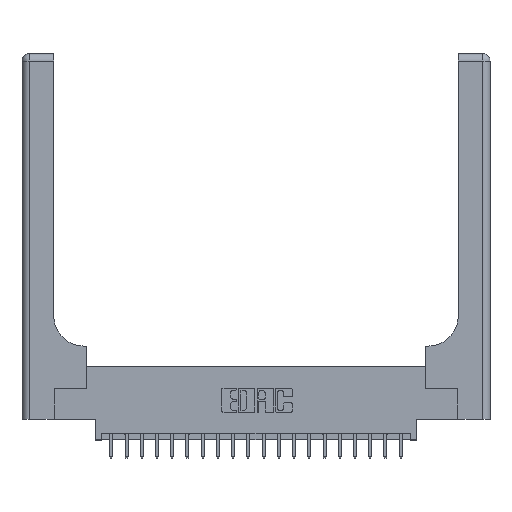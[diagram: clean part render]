
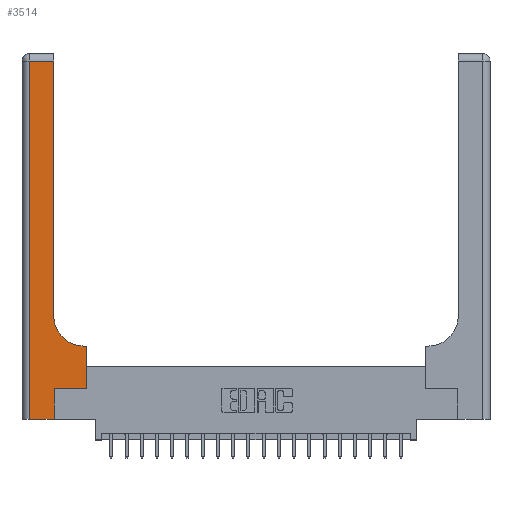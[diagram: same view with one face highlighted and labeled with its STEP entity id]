
A CAD part, top view. The second image highlights one B-rep face of the part: STEP entity #3514.
In plain terms, the highlighted planar face has unit normal (0, 0, 1).
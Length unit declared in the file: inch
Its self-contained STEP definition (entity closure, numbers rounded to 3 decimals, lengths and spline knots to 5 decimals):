
#363 = CARTESIAN_POINT ( 'NONE',  ( 0., 0., 0.37 ) ) ;
#433 = EDGE_CURVE ( 'NONE', #7438, #18347, #4337, .T. ) ;
#518 = EDGE_LOOP ( 'NONE', ( #19080, #19223, #4699, #2922, #15603, #11570, #15642, #14429, #13292 ) ) ;
#813 = EDGE_CURVE ( 'NONE', #16541, #18114, #10615, .T. ) ;
#1214 = CARTESIAN_POINT ( 'NONE',  ( 0.265, 0., 0.37 ) ) ;
#1371 = DIRECTION ( 'NONE',  ( 0., 0., -1. ) ) ;
#1857 = CARTESIAN_POINT ( 'NONE',  ( 0.528, 0.6, 0.37 ) ) ;
#1941 = EDGE_CURVE ( 'NONE', #14436, #12243, #16489, .T. ) ;
#1986 = EDGE_CURVE ( 'NONE', #7854, #16624, #10456, .T. ) ;
#1988 = AXIS2_PLACEMENT_3D ( 'NONE', #18352, #1371, #18024 ) ;
#2592 = PLANE ( 'NONE',  #16197 ) ;
#2777 = EDGE_CURVE ( 'NONE', #16624, #7438, #20082, .T. ) ;
#2892 = LINE ( 'NONE', #9523, #16131 ) ;
#2922 = ORIENTED_EDGE ( 'NONE', *, *, #813, .T. ) ;
#3074 = CARTESIAN_POINT ( 'NONE',  ( 0.26, 0.85, 0.37 ) ) ;
#3514 = ADVANCED_FACE ( 'NONE', ( #15956 ), #2592, .F. ) ;
#3978 = EDGE_CURVE ( 'NONE', #12243, #4757, #8069, .T. ) ;
#4292 = CARTESIAN_POINT ( 'NONE',  ( 0.06, 0., 0.37 ) ) ;
#4337 = LINE ( 'NONE', #7555, #20530 ) ;
#4699 = ORIENTED_EDGE ( 'NONE', *, *, #10388, .T. ) ;
#4757 = VERTEX_POINT ( 'NONE', #1857 ) ;
#5111 = LINE ( 'NONE', #18792, #20219 ) ;
#6352 = VECTOR ( 'NONE', #14799, 39.37008 ) ;
#7398 = LINE ( 'NONE', #17109, #15805 ) ;
#7438 = VERTEX_POINT ( 'NONE', #7890 ) ;
#7555 = CARTESIAN_POINT ( 'NONE',  ( 0., 2.94, 0.37 ) ) ;
#7854 = VERTEX_POINT ( 'NONE', #18119 ) ;
#7890 = CARTESIAN_POINT ( 'NONE',  ( 0.26, 2.94, 0.37 ) ) ;
#8069 = LINE ( 'NONE', #19318, #6352 ) ;
#8298 = EDGE_CURVE ( 'NONE', #18114, #14436, #7398, .T. ) ;
#8405 = VECTOR ( 'NONE', #13152, 39.37008 ) ;
#9523 = CARTESIAN_POINT ( 'NONE',  ( 0.26, 0.6, 0.37 ) ) ;
#9726 = CARTESIAN_POINT ( 'NONE',  ( 0.26, 3., 0.37 ) ) ;
#10388 = EDGE_CURVE ( 'NONE', #18347, #16541, #5111, .T. ) ;
#10391 = DIRECTION ( 'NONE',  ( 0., 1., 0. ) ) ;
#10456 = CIRCLE ( 'NONE', #1988, 0.25 ) ;
#10615 = LINE ( 'NONE', #363, #15276 ) ;
#11570 = ORIENTED_EDGE ( 'NONE', *, *, #1941, .T. ) ;
#12243 = VERTEX_POINT ( 'NONE', #19852 ) ;
#12337 = CARTESIAN_POINT ( 'NONE',  ( 0.265, 0.25, 0.37 ) ) ;
#12849 = DIRECTION ( 'NONE',  ( -1., 0., 0. ) ) ;
#13070 = DIRECTION ( 'NONE',  ( 1., 0., 0. ) ) ;
#13152 = DIRECTION ( 'NONE',  ( 0., 1., 0. ) ) ;
#13292 = ORIENTED_EDGE ( 'NONE', *, *, #1986, .T. ) ;
#13813 = DIRECTION ( 'NONE',  ( 1., 0., 0. ) ) ;
#13968 = VECTOR ( 'NONE', #13070, 39.37008 ) ;
#14429 = ORIENTED_EDGE ( 'NONE', *, *, #19047, .T. ) ;
#14436 = VERTEX_POINT ( 'NONE', #12337 ) ;
#14799 = DIRECTION ( 'NONE',  ( 0., 1., 0. ) ) ;
#14823 = DIRECTION ( 'NONE',  ( -1., 0., 0. ) ) ;
#15276 = VECTOR ( 'NONE', #13813, 39.37008 ) ;
#15603 = ORIENTED_EDGE ( 'NONE', *, *, #8298, .T. ) ;
#15642 = ORIENTED_EDGE ( 'NONE', *, *, #3978, .T. ) ;
#15805 = VECTOR ( 'NONE', #10391, 39.37008 ) ;
#15956 = FACE_OUTER_BOUND ( 'NONE', #518, .T. ) ;
#16131 = VECTOR ( 'NONE', #16246, 39.37008 ) ;
#16197 = AXIS2_PLACEMENT_3D ( 'NONE', #19894, #19156, #14823 ) ;
#16246 = DIRECTION ( 'NONE',  ( -1., 0., 0. ) ) ;
#16372 = CARTESIAN_POINT ( 'NONE',  ( 0.265, 0.25, 0.37 ) ) ;
#16489 = LINE ( 'NONE', #16372, #13968 ) ;
#16541 = VERTEX_POINT ( 'NONE', #4292 ) ;
#16624 = VERTEX_POINT ( 'NONE', #3074 ) ;
#17109 = CARTESIAN_POINT ( 'NONE',  ( 0.265, 0., 0.37 ) ) ;
#18024 = DIRECTION ( 'NONE',  ( 1., 0., 0. ) ) ;
#18114 = VERTEX_POINT ( 'NONE', #1214 ) ;
#18119 = CARTESIAN_POINT ( 'NONE',  ( 0.51, 0.6, 0.37 ) ) ;
#18347 = VERTEX_POINT ( 'NONE', #19171 ) ;
#18352 = CARTESIAN_POINT ( 'NONE',  ( 0.51, 0.85, 0.37 ) ) ;
#18574 = DIRECTION ( 'NONE',  ( 0., -1., 0. ) ) ;
#18792 = CARTESIAN_POINT ( 'NONE',  ( 0.06, 3., 0.37 ) ) ;
#19047 = EDGE_CURVE ( 'NONE', #4757, #7854, #2892, .T. ) ;
#19080 = ORIENTED_EDGE ( 'NONE', *, *, #2777, .T. ) ;
#19156 = DIRECTION ( 'NONE',  ( 0., 0., -1. ) ) ;
#19171 = CARTESIAN_POINT ( 'NONE',  ( 0.06, 2.94, 0.37 ) ) ;
#19223 = ORIENTED_EDGE ( 'NONE', *, *, #433, .T. ) ;
#19318 = CARTESIAN_POINT ( 'NONE',  ( 0.528, 0.25, 0.37 ) ) ;
#19852 = CARTESIAN_POINT ( 'NONE',  ( 0.528, 0.25, 0.37 ) ) ;
#19894 = CARTESIAN_POINT ( 'NONE',  ( 0., 3., 0.37 ) ) ;
#20082 = LINE ( 'NONE', #9726, #8405 ) ;
#20219 = VECTOR ( 'NONE', #18574, 39.37008 ) ;
#20530 = VECTOR ( 'NONE', #12849, 39.37008 ) ;
